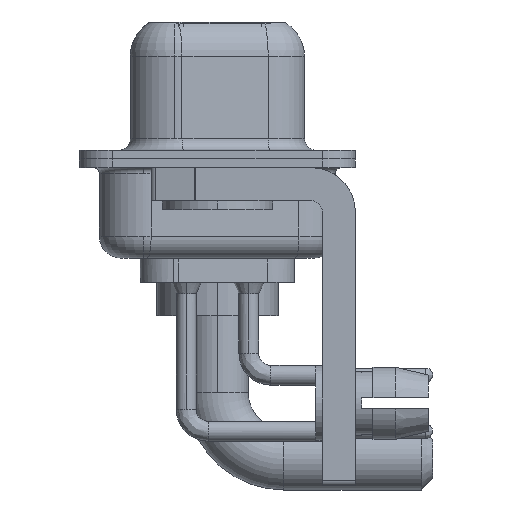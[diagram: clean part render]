
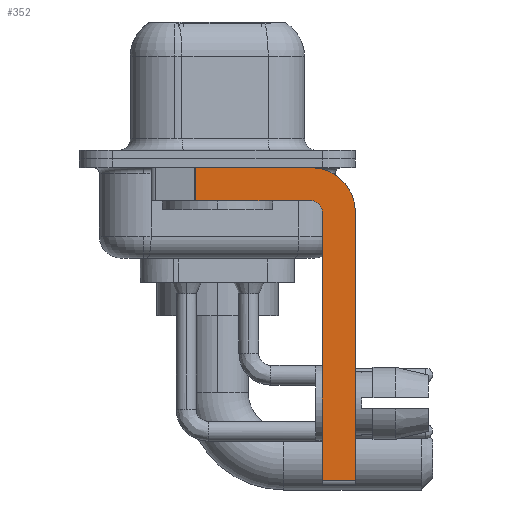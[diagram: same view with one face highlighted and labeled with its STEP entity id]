
A CAD part, left-side view. The second image highlights one B-rep face of the part: STEP entity #352.
In plain terms, the highlighted planar face has unit normal (-1, 0, 0).
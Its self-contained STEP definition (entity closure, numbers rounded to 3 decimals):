
#37 = EDGE_CURVE ( 'NONE', #579, #23496, #7321, .T. ) ;
#254 = VERTEX_POINT ( 'NONE', #12130 ) ;
#352 = ADVANCED_FACE ( 'NONE', ( #18373 ), #14849, .F. ) ;
#579 = VERTEX_POINT ( 'NONE', #638 ) ;
#638 = CARTESIAN_POINT ( 'NONE',  ( -2.9, 0.978, -0.4 ) ) ;
#648 = ORIENTED_EDGE ( 'NONE', *, *, #2465, .F. ) ;
#936 = EDGE_CURVE ( 'NONE', #24643, #18669, #1874, .T. ) ;
#1392 = ORIENTED_EDGE ( 'NONE', *, *, #3663, .T. ) ;
#1872 = CIRCLE ( 'NONE', #10363, 0.5 ) ;
#1874 = LINE ( 'NONE', #3901, #14008 ) ;
#2210 = LINE ( 'NONE', #11960, #24016 ) ;
#2217 = ORIENTED_EDGE ( 'NONE', *, *, #2336, .F. ) ;
#2336 = EDGE_CURVE ( 'NONE', #11162, #24643, #18328, .T. ) ;
#2465 = EDGE_CURVE ( 'NONE', #15361, #254, #1872, .T. ) ;
#3134 = LINE ( 'NONE', #17060, #20764 ) ;
#3663 = EDGE_CURVE ( 'NONE', #7650, #18669, #22897, .T. ) ;
#3731 = DIRECTION ( 'NONE',  ( 0., -1., 0. ) ) ;
#3901 = CARTESIAN_POINT ( 'NONE',  ( -2.9, -6.25, -2.4 ) ) ;
#4841 = ORIENTED_EDGE ( 'NONE', *, *, #37, .T. ) ;
#5073 = DIRECTION ( 'NONE',  ( 1., 0., 0. ) ) ;
#6192 = AXIS2_PLACEMENT_3D ( 'NONE', #23904, #6563, #16061 ) ;
#6563 = DIRECTION ( 'NONE',  ( 1., 0., 0. ) ) ;
#6685 = DIRECTION ( 'NONE',  ( 0., 0., 1. ) ) ;
#6882 = CARTESIAN_POINT ( 'NONE',  ( -2.9, -4.75, -2.4 ) ) ;
#6904 = VECTOR ( 'NONE', #14960, 1000. ) ;
#7194 = CARTESIAN_POINT ( 'NONE',  ( -2.9, -4.25, -14.55 ) ) ;
#7299 = DIRECTION ( 'NONE',  ( 0., 0., 1. ) ) ;
#7321 = LINE ( 'NONE', #8720, #8693 ) ;
#7650 = VERTEX_POINT ( 'NONE', #24759 ) ;
#7992 = ORIENTED_EDGE ( 'NONE', *, *, #23237, .F. ) ;
#8140 = CARTESIAN_POINT ( 'NONE',  ( -2.9, 0.978, -1.9 ) ) ;
#8693 = VECTOR ( 'NONE', #24435, 1000. ) ;
#8720 = CARTESIAN_POINT ( 'NONE',  ( -2.9, 0.978, -1.9 ) ) ;
#10363 = AXIS2_PLACEMENT_3D ( 'NONE', #21997, #24035, #6685 ) ;
#10723 = CARTESIAN_POINT ( 'NONE',  ( -2.9, -6.25, -2.4 ) ) ;
#11162 = VERTEX_POINT ( 'NONE', #15530 ) ;
#11358 = ORIENTED_EDGE ( 'NONE', *, *, #21238, .F. ) ;
#11393 = VECTOR ( 'NONE', #18598, 1000. ) ;
#11960 = CARTESIAN_POINT ( 'NONE',  ( -2.9, 3., -0.4 ) ) ;
#12130 = CARTESIAN_POINT ( 'NONE',  ( -2.9, -4.25, -1.9 ) ) ;
#14008 = VECTOR ( 'NONE', #17323, 1000. ) ;
#14224 = ORIENTED_EDGE ( 'NONE', *, *, #936, .F. ) ;
#14363 = AXIS2_PLACEMENT_3D ( 'NONE', #16854, #5073, #14599 ) ;
#14599 = DIRECTION ( 'NONE',  ( 0., 0., -1. ) ) ;
#14619 = CARTESIAN_POINT ( 'NONE',  ( -2.9, -6.25, -14.55 ) ) ;
#14849 = PLANE ( 'NONE',  #14363 ) ;
#14960 = DIRECTION ( 'NONE',  ( 0., -1., 0. ) ) ;
#15361 = VERTEX_POINT ( 'NONE', #6882 ) ;
#15530 = CARTESIAN_POINT ( 'NONE',  ( -2.9, -4.25, -0.4 ) ) ;
#16061 = DIRECTION ( 'NONE',  ( 0., 0., -1. ) ) ;
#16683 = ORIENTED_EDGE ( 'NONE', *, *, #19452, .F. ) ;
#16854 = CARTESIAN_POINT ( 'NONE',  ( -2.9, -4.25, -2.4 ) ) ;
#16959 = LINE ( 'NONE', #17087, #11393 ) ;
#17060 = CARTESIAN_POINT ( 'NONE',  ( -2.9, -4.75, -14.8 ) ) ;
#17087 = CARTESIAN_POINT ( 'NONE',  ( -2.9, -4.25, -1.9 ) ) ;
#17323 = DIRECTION ( 'NONE',  ( 0., 0., -1. ) ) ;
#18328 = CIRCLE ( 'NONE', #6192, 2. ) ;
#18373 = FACE_OUTER_BOUND ( 'NONE', #21529, .T. ) ;
#18598 = DIRECTION ( 'NONE',  ( 0., 1., 0. ) ) ;
#18669 = VERTEX_POINT ( 'NONE', #14619 ) ;
#19452 = EDGE_CURVE ( 'NONE', #254, #23496, #16959, .T. ) ;
#20764 = VECTOR ( 'NONE', #7299, 1000. ) ;
#21238 = EDGE_CURVE ( 'NONE', #7650, #15361, #3134, .T. ) ;
#21529 = EDGE_LOOP ( 'NONE', ( #7992, #4841, #16683, #648, #11358, #1392, #14224, #2217 ) ) ;
#21997 = CARTESIAN_POINT ( 'NONE',  ( -2.9, -4.25, -2.4 ) ) ;
#22897 = LINE ( 'NONE', #7194, #6904 ) ;
#23237 = EDGE_CURVE ( 'NONE', #579, #11162, #2210, .T. ) ;
#23496 = VERTEX_POINT ( 'NONE', #8140 ) ;
#23904 = CARTESIAN_POINT ( 'NONE',  ( -2.9, -4.25, -2.4 ) ) ;
#24016 = VECTOR ( 'NONE', #3731, 1000. ) ;
#24035 = DIRECTION ( 'NONE',  ( -1., 0., 0. ) ) ;
#24435 = DIRECTION ( 'NONE',  ( 0., 0., -1. ) ) ;
#24643 = VERTEX_POINT ( 'NONE', #10723 ) ;
#24759 = CARTESIAN_POINT ( 'NONE',  ( -2.9, -4.75, -14.55 ) ) ;
